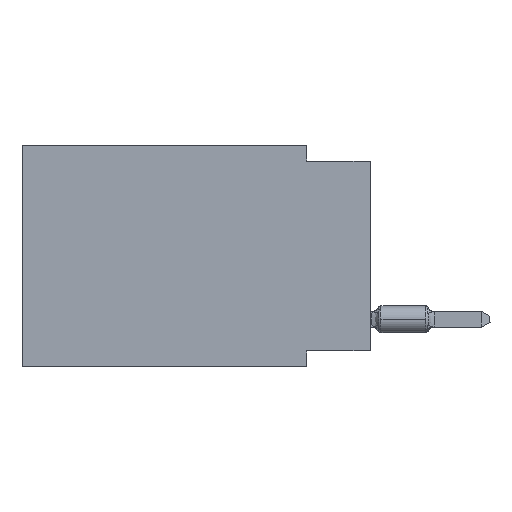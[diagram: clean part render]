
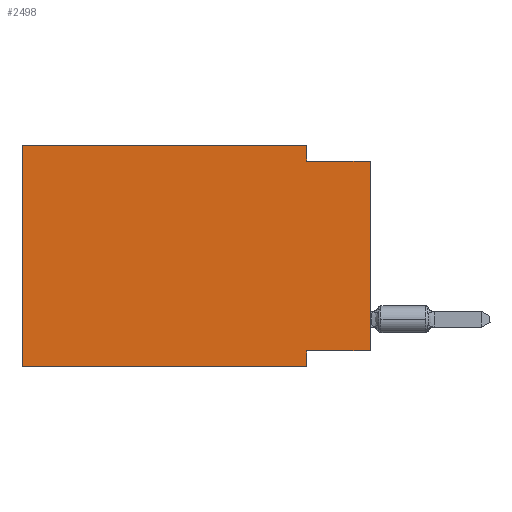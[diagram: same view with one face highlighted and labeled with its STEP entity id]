
A CAD part, left-side view. The second image highlights one B-rep face of the part: STEP entity #2498.
In plain terms, the highlighted planar face has unit normal (-1, 0, 0).
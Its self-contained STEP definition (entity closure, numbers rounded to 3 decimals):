
#700 = VECTOR ( 'NONE', #37280, 1000. ) ;
#1001 = EDGE_CURVE ( 'NONE', #9298, #35977, #45091, .T. ) ;
#1247 = CARTESIAN_POINT ( 'NONE',  ( 0., 2.54, -8.255 ) ) ;
#1882 = DIRECTION ( 'NONE',  ( 0., 0., -1. ) ) ;
#1933 = EDGE_CURVE ( 'NONE', #21161, #22152, #26176, .T. ) ;
#2058 = CARTESIAN_POINT ( 'NONE',  ( 0., 0., 0. ) ) ;
#2498 = ADVANCED_FACE ( 'NONE', ( #41480 ), #30923, .F. ) ;
#3881 = LINE ( 'NONE', #30037, #28911 ) ;
#5527 = VERTEX_POINT ( 'NONE', #25230 ) ;
#5935 = ORIENTED_EDGE ( 'NONE', *, *, #27816, .F. ) ;
#7004 = DIRECTION ( 'NONE',  ( 0., -1., 0. ) ) ;
#7272 = DIRECTION ( 'NONE',  ( 0., 0., 1. ) ) ;
#7831 = VECTOR ( 'NONE', #7957, 1000. ) ;
#7957 = DIRECTION ( 'NONE',  ( 0., -1., 0. ) ) ;
#9298 = VERTEX_POINT ( 'NONE', #45998 ) ;
#9491 = DIRECTION ( 'NONE',  ( 0., 0., 1. ) ) ;
#10521 = ORIENTED_EDGE ( 'NONE', *, *, #19725, .T. ) ;
#10611 = CARTESIAN_POINT ( 'NONE',  ( 0., 13.97, 0. ) ) ;
#10876 = VECTOR ( 'NONE', #12222, 1000. ) ;
#11619 = VERTEX_POINT ( 'NONE', #23906 ) ;
#12061 = LINE ( 'NONE', #15188, #700 ) ;
#12222 = DIRECTION ( 'NONE',  ( 0., 0., -1. ) ) ;
#14029 = CARTESIAN_POINT ( 'NONE',  ( 0., 0., -0.635 ) ) ;
#15188 = CARTESIAN_POINT ( 'NONE',  ( 0., 2.54, 0. ) ) ;
#15504 = VECTOR ( 'NONE', #18356, 1000. ) ;
#15802 = DIRECTION ( 'NONE',  ( 0., 1., 0. ) ) ;
#15983 = EDGE_LOOP ( 'NONE', ( #26356, #32407, #21852, #17717, #5935, #10521, #25303, #26999 ) ) ;
#17717 = ORIENTED_EDGE ( 'NONE', *, *, #1933, .F. ) ;
#17947 = VERTEX_POINT ( 'NONE', #14029 ) ;
#18294 = LINE ( 'NONE', #40153, #27055 ) ;
#18356 = DIRECTION ( 'NONE',  ( 0., -1., 0. ) ) ;
#18466 = VECTOR ( 'NONE', #15802, 1000. ) ;
#19725 = EDGE_CURVE ( 'NONE', #11619, #5527, #3881, .T. ) ;
#21161 = VERTEX_POINT ( 'NONE', #10611 ) ;
#21852 = ORIENTED_EDGE ( 'NONE', *, *, #34823, .F. ) ;
#22152 = VERTEX_POINT ( 'NONE', #30580 ) ;
#22363 = CARTESIAN_POINT ( 'NONE',  ( 0., 2.54, -0.635 ) ) ;
#23906 = CARTESIAN_POINT ( 'NONE',  ( 0., 13.97, -8.89 ) ) ;
#25230 = CARTESIAN_POINT ( 'NONE',  ( 0., 2.54, -8.89 ) ) ;
#25303 = ORIENTED_EDGE ( 'NONE', *, *, #27111, .F. ) ;
#25565 = LINE ( 'NONE', #36620, #15504 ) ;
#26176 = LINE ( 'NONE', #40836, #7831 ) ;
#26356 = ORIENTED_EDGE ( 'NONE', *, *, #29687, .T. ) ;
#26632 = LINE ( 'NONE', #27102, #10876 ) ;
#26999 = ORIENTED_EDGE ( 'NONE', *, *, #1001, .F. ) ;
#27055 = VECTOR ( 'NONE', #7272, 1000. ) ;
#27102 = CARTESIAN_POINT ( 'NONE',  ( 0., 2.54, -8.89 ) ) ;
#27111 = EDGE_CURVE ( 'NONE', #35977, #5527, #26632, .T. ) ;
#27312 = CARTESIAN_POINT ( 'NONE',  ( 0., 13.97, 0. ) ) ;
#27487 = EDGE_CURVE ( 'NONE', #39862, #17947, #25565, .T. ) ;
#27803 = VECTOR ( 'NONE', #9491, 1000. ) ;
#27816 = EDGE_CURVE ( 'NONE', #11619, #21161, #18294, .T. ) ;
#28911 = VECTOR ( 'NONE', #7004, 1000. ) ;
#29687 = EDGE_CURVE ( 'NONE', #9298, #17947, #34955, .T. ) ;
#30037 = CARTESIAN_POINT ( 'NONE',  ( 0., 13.97, -8.89 ) ) ;
#30580 = CARTESIAN_POINT ( 'NONE',  ( 0., 2.54, 0. ) ) ;
#30923 = PLANE ( 'NONE',  #31641 ) ;
#31641 = AXIS2_PLACEMENT_3D ( 'NONE', #27312, #34764, #1882 ) ;
#32407 = ORIENTED_EDGE ( 'NONE', *, *, #27487, .F. ) ;
#33361 = CARTESIAN_POINT ( 'NONE',  ( 0., 0., -8.255 ) ) ;
#34764 = DIRECTION ( 'NONE',  ( 1., 0., 0. ) ) ;
#34823 = EDGE_CURVE ( 'NONE', #22152, #39862, #12061, .T. ) ;
#34955 = LINE ( 'NONE', #2058, #27803 ) ;
#35977 = VERTEX_POINT ( 'NONE', #1247 ) ;
#36620 = CARTESIAN_POINT ( 'NONE',  ( 0., 0., -0.635 ) ) ;
#37280 = DIRECTION ( 'NONE',  ( 0., 0., -1. ) ) ;
#39862 = VERTEX_POINT ( 'NONE', #22363 ) ;
#40153 = CARTESIAN_POINT ( 'NONE',  ( 0., 13.97, 0. ) ) ;
#40836 = CARTESIAN_POINT ( 'NONE',  ( 0., 13.97, 0. ) ) ;
#41480 = FACE_OUTER_BOUND ( 'NONE', #15983, .T. ) ;
#45091 = LINE ( 'NONE', #33361, #18466 ) ;
#45998 = CARTESIAN_POINT ( 'NONE',  ( 0., 0., -8.255 ) ) ;
